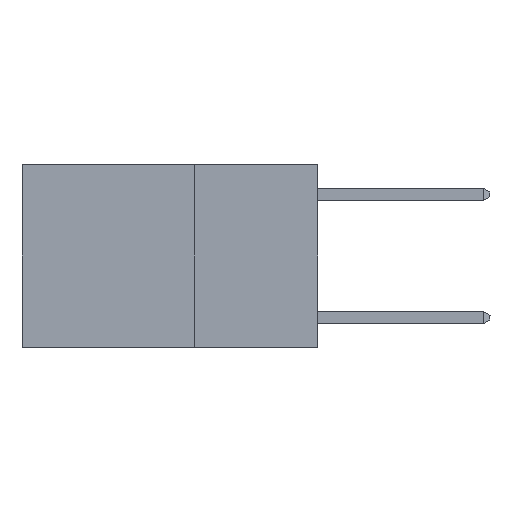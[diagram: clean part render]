
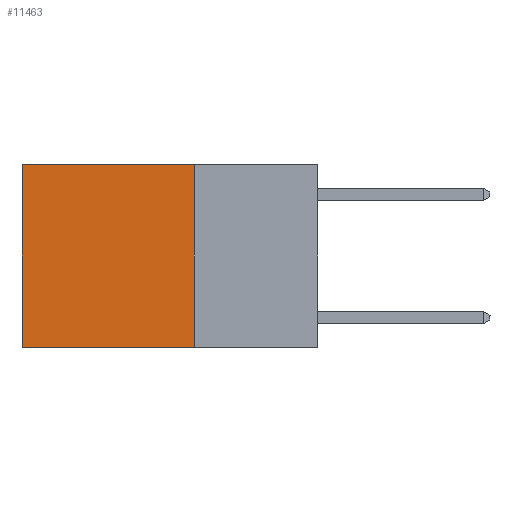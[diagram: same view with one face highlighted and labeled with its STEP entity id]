
A CAD part, left-side view. The second image highlights one B-rep face of the part: STEP entity #11463.
In plain terms, the highlighted planar face has unit normal (-1, 0, 0).
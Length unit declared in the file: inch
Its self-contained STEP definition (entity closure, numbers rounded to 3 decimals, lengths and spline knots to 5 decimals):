
#147 = ORIENTED_EDGE ( 'NONE', *, *, #5197, .T. ) ;
#152 = CARTESIAN_POINT ( 'NONE',  ( 0.2625, 0.25, -0.37 ) ) ;
#312 = ORIENTED_EDGE ( 'NONE', *, *, #12733, .T. ) ;
#582 = DIRECTION ( 'NONE',  ( 0., 1., 0. ) ) ;
#592 = LINE ( 'NONE', #23016, #13541 ) ;
#800 = CARTESIAN_POINT ( 'NONE',  ( 0.2625, 0.25, 0. ) ) ;
#1088 = DIRECTION ( 'NONE',  ( 0., 0., -1. ) ) ;
#1498 = FACE_OUTER_BOUND ( 'NONE', #3787, .T. ) ;
#1698 = ORIENTED_EDGE ( 'NONE', *, *, #5021, .F. ) ;
#3137 = DIRECTION ( 'NONE',  ( 1., 0., 0. ) ) ;
#3571 = ORIENTED_EDGE ( 'NONE', *, *, #8465, .F. ) ;
#3787 = EDGE_LOOP ( 'NONE', ( #312, #1698, #3571, #147 ) ) ;
#5021 = EDGE_CURVE ( 'NONE', #5626, #6276, #10105, .T. ) ;
#5197 = EDGE_CURVE ( 'NONE', #15038, #24671, #17570, .T. ) ;
#5626 = VERTEX_POINT ( 'NONE', #152 ) ;
#6276 = VERTEX_POINT ( 'NONE', #25654 ) ;
#8080 = CARTESIAN_POINT ( 'NONE',  ( 0.2625, 0.6, 0. ) ) ;
#8465 = EDGE_CURVE ( 'NONE', #15038, #5626, #592, .T. ) ;
#10105 = LINE ( 'NONE', #10228, #25640 ) ;
#10228 = CARTESIAN_POINT ( 'NONE',  ( 0.2625, 0.25, -0.37 ) ) ;
#11152 = CARTESIAN_POINT ( 'NONE',  ( 0.2625, 0.25, 0. ) ) ;
#11463 = ADVANCED_FACE ( 'NONE', ( #1498 ), #26100, .F. ) ;
#12290 = DIRECTION ( 'NONE',  ( 0., 1., 0. ) ) ;
#12733 = EDGE_CURVE ( 'NONE', #24671, #6276, #15402, .T. ) ;
#13541 = VECTOR ( 'NONE', #18945, 39.37008 ) ;
#14356 = VECTOR ( 'NONE', #582, 39.37008 ) ;
#14661 = VECTOR ( 'NONE', #16059, 39.37008 ) ;
#15038 = VERTEX_POINT ( 'NONE', #800 ) ;
#15402 = LINE ( 'NONE', #23694, #14661 ) ;
#16059 = DIRECTION ( 'NONE',  ( 0., 0., -1. ) ) ;
#17570 = LINE ( 'NONE', #11152, #14356 ) ;
#17734 = AXIS2_PLACEMENT_3D ( 'NONE', #18077, #3137, #1088 ) ;
#18077 = CARTESIAN_POINT ( 'NONE',  ( 0.2625, 0.25, 0. ) ) ;
#18945 = DIRECTION ( 'NONE',  ( 0., 0., -1. ) ) ;
#23016 = CARTESIAN_POINT ( 'NONE',  ( 0.2625, 0.25, 0. ) ) ;
#23694 = CARTESIAN_POINT ( 'NONE',  ( 0.2625, 0.6, 0. ) ) ;
#24671 = VERTEX_POINT ( 'NONE', #8080 ) ;
#25640 = VECTOR ( 'NONE', #12290, 39.37008 ) ;
#25654 = CARTESIAN_POINT ( 'NONE',  ( 0.2625, 0.6, -0.37 ) ) ;
#26100 = PLANE ( 'NONE',  #17734 ) ;
